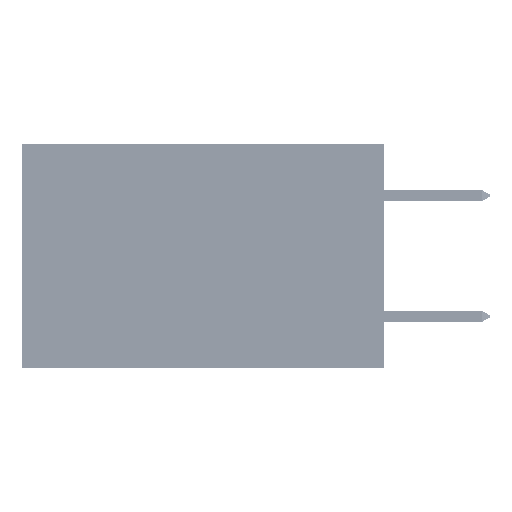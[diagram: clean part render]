
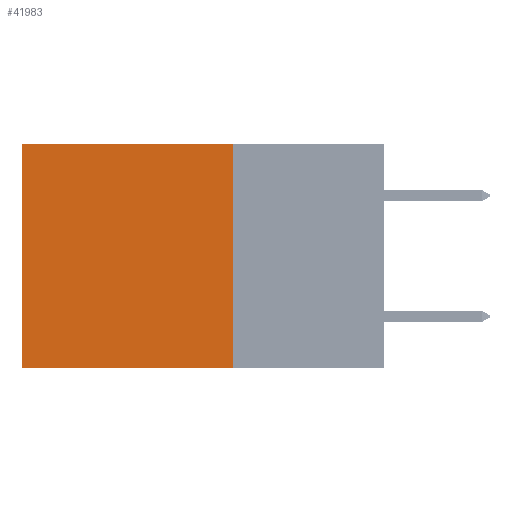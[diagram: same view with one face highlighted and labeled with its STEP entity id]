
A CAD part, left-side view. The second image highlights one B-rep face of the part: STEP entity #41983.
In plain terms, the highlighted planar face has unit normal (-1, 0, 0).
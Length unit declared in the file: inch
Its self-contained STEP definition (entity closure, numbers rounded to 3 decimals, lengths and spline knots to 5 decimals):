
#882 = CARTESIAN_POINT ( 'NONE',  ( 0.2875, 0.25, 0. ) ) ;
#1471 = VERTEX_POINT ( 'NONE', #882 ) ;
#1524 = CARTESIAN_POINT ( 'NONE',  ( 0.2875, 0.25, 0. ) ) ;
#2522 = CARTESIAN_POINT ( 'NONE',  ( 0.2875, 0.25, -0.37 ) ) ;
#4911 = VERTEX_POINT ( 'NONE', #8591 ) ;
#4951 = LINE ( 'NONE', #43912, #45889 ) ;
#5893 = CARTESIAN_POINT ( 'NONE',  ( 0.2875, 0.6, 0. ) ) ;
#6171 = ORIENTED_EDGE ( 'NONE', *, *, #8729, .T. ) ;
#8591 = CARTESIAN_POINT ( 'NONE',  ( 0.2875, 0.6, -0.37 ) ) ;
#8729 = EDGE_CURVE ( 'NONE', #37000, #4911, #4951, .T. ) ;
#9669 = DIRECTION ( 'NONE',  ( 1., 0., 0. ) ) ;
#13097 = DIRECTION ( 'NONE',  ( 0., 1., 0. ) ) ;
#13646 = DIRECTION ( 'NONE',  ( 0., 0., -1. ) ) ;
#15133 = ORIENTED_EDGE ( 'NONE', *, *, #18596, .T. ) ;
#18410 = DIRECTION ( 'NONE',  ( 0., 1., 0. ) ) ;
#18596 = EDGE_CURVE ( 'NONE', #1471, #37000, #37487, .T. ) ;
#22459 = VECTOR ( 'NONE', #18410, 39.37008 ) ;
#23445 = FACE_OUTER_BOUND ( 'NONE', #43415, .T. ) ;
#25202 = CARTESIAN_POINT ( 'NONE',  ( 0.2875, 0.25, 0. ) ) ;
#25547 = VECTOR ( 'NONE', #33051, 39.37008 ) ;
#25583 = VERTEX_POINT ( 'NONE', #40125 ) ;
#28719 = LINE ( 'NONE', #2522, #22459 ) ;
#28918 = PLANE ( 'NONE',  #50729 ) ;
#33051 = DIRECTION ( 'NONE',  ( 0., 0., -1. ) ) ;
#35761 = DIRECTION ( 'NONE',  ( 0., 0., -1. ) ) ;
#37000 = VERTEX_POINT ( 'NONE', #5893 ) ;
#37487 = LINE ( 'NONE', #44138, #41220 ) ;
#40125 = CARTESIAN_POINT ( 'NONE',  ( 0.2875, 0.25, -0.37 ) ) ;
#41134 = LINE ( 'NONE', #25202, #25547 ) ;
#41220 = VECTOR ( 'NONE', #13097, 39.37008 ) ;
#41464 = ORIENTED_EDGE ( 'NONE', *, *, #45223, .F. ) ;
#41983 = ADVANCED_FACE ( 'NONE', ( #23445 ), #28918, .F. ) ;
#43415 = EDGE_LOOP ( 'NONE', ( #6171, #41464, #44482, #15133 ) ) ;
#43912 = CARTESIAN_POINT ( 'NONE',  ( 0.2875, 0.6, 0. ) ) ;
#44138 = CARTESIAN_POINT ( 'NONE',  ( 0.2875, 0.25, 0. ) ) ;
#44482 = ORIENTED_EDGE ( 'NONE', *, *, #48941, .F. ) ;
#45223 = EDGE_CURVE ( 'NONE', #25583, #4911, #28719, .T. ) ;
#45889 = VECTOR ( 'NONE', #35761, 39.37008 ) ;
#48941 = EDGE_CURVE ( 'NONE', #1471, #25583, #41134, .T. ) ;
#50729 = AXIS2_PLACEMENT_3D ( 'NONE', #1524, #9669, #13646 ) ;
